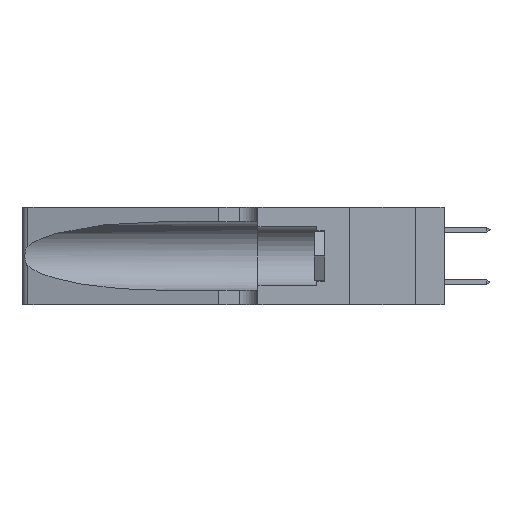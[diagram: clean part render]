
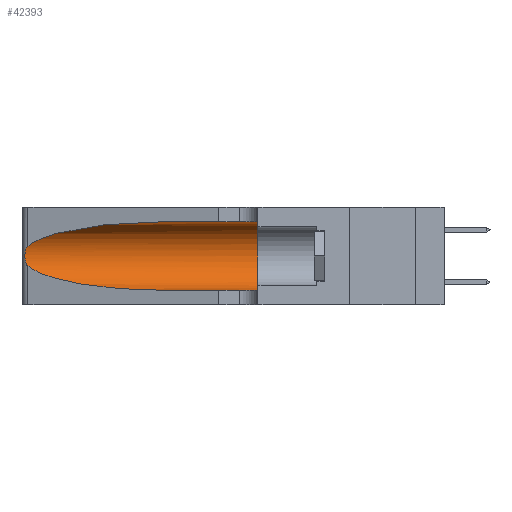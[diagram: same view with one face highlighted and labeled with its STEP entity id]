
A CAD part, left-side view. The second image highlights one B-rep face of the part: STEP entity #42393.
In plain terms, the highlighted cylindrical face has radius 3.308 mm (diameter 6.617 mm), a partial arc.
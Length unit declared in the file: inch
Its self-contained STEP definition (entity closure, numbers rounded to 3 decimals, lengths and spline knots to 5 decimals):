
#1410 = CARTESIAN_POINT ( 'NONE',  ( 0.26075, 1.23896, 0.178 ) ) ;
#1549 = CARTESIAN_POINT ( 'NONE',  ( 0.25854, 1.2359, 0.20912 ) ) ;
#2740 =( BOUNDED_CURVE ( )  B_SPLINE_CURVE ( 3, ( #5531, #25477, #35617, #6346 ),
 .UNSPECIFIED., .F., .F. ) 
 B_SPLINE_CURVE_WITH_KNOTS ( ( 4, 4 ),
 ( 1.5708, 2.84003 ),
 .UNSPECIFIED. ) 
 CURVE ( )  GEOMETRIC_REPRESENTATION_ITEM ( )  RATIONAL_B_SPLINE_CURVE ( ( 1., 0.87, 0.87, 1. ) ) 
 REPRESENTATION_ITEM ( '' )  );
#4674 = CARTESIAN_POINT ( 'NONE',  ( 0.25789, 1.23486, 0.15765 ) ) ;
#5241 = DIRECTION ( 'NONE',  ( 0., -1., 0. ) ) ;
#5279 = EDGE_CURVE ( 'NONE', #29261, #35275, #19362, .T. ) ;
#5531 = CARTESIAN_POINT ( 'NONE',  ( 0.1305, 0.72297, 0.31525 ) ) ;
#5534 = CARTESIAN_POINT ( 'NONE',  ( 0.1305, 1.61858, 0.185 ) ) ;
#6346 = CARTESIAN_POINT ( 'NONE',  ( 0.25487, 1.22718, 0.22369 ) ) ;
#7813 = CARTESIAN_POINT ( 'NONE',  ( 0.25856, 1.23593, 0.16098 ) ) ;
#8115 = CARTESIAN_POINT ( 'NONE',  ( 0.25555, 1.22994, 0.2215 ) ) ;
#9507 = ORIENTED_EDGE ( 'NONE', *, *, #23897, .T. ) ;
#10848 = B_SPLINE_CURVE_WITH_KNOTS ( 'NONE', 3,
 ( #21062, #8115, #34177, #40543, #1549, #24345, #31143, #1410, #24491, #7813, #4674, #30851, #27969, #20884 ),
 .UNSPECIFIED., .F., .F.,
 ( 4, 2, 2, 2, 2, 2, 4 ),
 ( 0., 0.00027, 0.00053, 0.00107, 0.0016, 0.00187, 0.00214 ),
 .UNSPECIFIED. ) ;
#11268 = DIRECTION ( 'NONE',  ( 0., 1., 0. ) ) ;
#11729 = CARTESIAN_POINT ( 'NONE',  ( 0.25487, 1.22718, 0.22369 ) ) ;
#13316 = EDGE_CURVE ( 'NONE', #35985, #35275, #42242, .T. ) ;
#14075 = CARTESIAN_POINT ( 'NONE',  ( 0.1305, 0.35, 0.05475 ) ) ;
#14426 = DIRECTION ( 'NONE',  ( 0., 0., 1. ) ) ;
#15005 = CARTESIAN_POINT ( 'NONE',  ( 0.1305, 1.61858, 0.31525 ) ) ;
#16209 = AXIS2_PLACEMENT_3D ( 'NONE', #5534, #18297, #28076 ) ;
#16345 = CARTESIAN_POINT ( 'NONE',  ( 0.1305, 0.72297, 0.05475 ) ) ;
#17850 = ORIENTED_EDGE ( 'NONE', *, *, #13316, .F. ) ;
#17932 = DIRECTION ( 'NONE',  ( 0., -1., 0. ) ) ;
#18297 = DIRECTION ( 'NONE',  ( 0., -1., 0. ) ) ;
#19362 = LINE ( 'NONE', #27725, #31795 ) ;
#20579 = CARTESIAN_POINT ( 'NONE',  ( 0.25487, 1.22718, 0.14631 ) ) ;
#20792 = ORIENTED_EDGE ( 'NONE', *, *, #36692, .T. ) ;
#20884 = CARTESIAN_POINT ( 'NONE',  ( 0.25487, 1.22718, 0.14631 ) ) ;
#21057 = AXIS2_PLACEMENT_3D ( 'NONE', #34164, #11268, #14426 ) ;
#21062 = CARTESIAN_POINT ( 'NONE',  ( 0.25487, 1.22718, 0.22369 ) ) ;
#21414 = CARTESIAN_POINT ( 'NONE',  ( 0.1305, 0.72297, 0.31525 ) ) ;
#21697 = CARTESIAN_POINT ( 'NONE',  ( 0.2373, 1.15595, 0.08982 ) ) ;
#22472 =( BOUNDED_CURVE ( )  B_SPLINE_CURVE ( 3, ( #41901, #21697, #38868, #16345 ),
 .UNSPECIFIED., .F., .F. ) 
 B_SPLINE_CURVE_WITH_KNOTS ( ( 4, 4 ),
 ( 3.44316, 4.71239 ),
 .UNSPECIFIED. ) 
 CURVE ( )  GEOMETRIC_REPRESENTATION_ITEM ( )  RATIONAL_B_SPLINE_CURVE ( ( 1., 0.87, 0.87, 1. ) ) 
 REPRESENTATION_ITEM ( '' )  );
#23897 = EDGE_CURVE ( 'NONE', #36550, #29261, #22472, .T. ) ;
#24345 = CARTESIAN_POINT ( 'NONE',  ( 0.26018, 1.23835, 0.19895 ) ) ;
#24491 = CARTESIAN_POINT ( 'NONE',  ( 0.26017, 1.23833, 0.17102 ) ) ;
#24804 = ORIENTED_EDGE ( 'NONE', *, *, #28854, .F. ) ;
#25477 = CARTESIAN_POINT ( 'NONE',  ( 0.18966, 0.96281, 0.31525 ) ) ;
#27725 = CARTESIAN_POINT ( 'NONE',  ( 0.1305, 1.61858, 0.05475 ) ) ;
#27969 = CARTESIAN_POINT ( 'NONE',  ( 0.25555, 1.22993, 0.14849 ) ) ;
#28076 = DIRECTION ( 'NONE',  ( 0., 0., -1. ) ) ;
#28854 = EDGE_CURVE ( 'NONE', #37371, #35985, #39731, .T. ) ;
#29261 = VERTEX_POINT ( 'NONE', #34269 ) ;
#29426 = CARTESIAN_POINT ( 'NONE',  ( 0.1305, 0.35, 0.31525 ) ) ;
#29814 = EDGE_CURVE ( 'NONE', #37371, #37535, #2740, .T. ) ;
#30851 = CARTESIAN_POINT ( 'NONE',  ( 0.25639, 1.23186, 0.15144 ) ) ;
#30926 = VECTOR ( 'NONE', #5241, 39.37008 ) ;
#31143 = CARTESIAN_POINT ( 'NONE',  ( 0.26075, 1.23896, 0.19203 ) ) ;
#31795 = VECTOR ( 'NONE', #17932, 39.37008 ) ;
#34164 = CARTESIAN_POINT ( 'NONE',  ( 0.1305, 0.35, 0.185 ) ) ;
#34177 = CARTESIAN_POINT ( 'NONE',  ( 0.25639, 1.23184, 0.21858 ) ) ;
#34269 = CARTESIAN_POINT ( 'NONE',  ( 0.1305, 0.72297, 0.05475 ) ) ;
#34827 = ORIENTED_EDGE ( 'NONE', *, *, #29814, .T. ) ;
#35275 = VERTEX_POINT ( 'NONE', #14075 ) ;
#35617 = CARTESIAN_POINT ( 'NONE',  ( 0.2373, 1.15595, 0.28018 ) ) ;
#35985 = VERTEX_POINT ( 'NONE', #29426 ) ;
#36550 = VERTEX_POINT ( 'NONE', #20579 ) ;
#36692 = EDGE_CURVE ( 'NONE', #37535, #36550, #10848, .T. ) ;
#36757 = EDGE_LOOP ( 'NONE', ( #34827, #20792, #9507, #40102, #17850, #24804 ) ) ;
#36830 = CYLINDRICAL_SURFACE ( 'NONE', #16209, 0.13025 ) ;
#37371 = VERTEX_POINT ( 'NONE', #21414 ) ;
#37535 = VERTEX_POINT ( 'NONE', #11729 ) ;
#38868 = CARTESIAN_POINT ( 'NONE',  ( 0.18966, 0.96281, 0.05475 ) ) ;
#39731 = LINE ( 'NONE', #15005, #30926 ) ;
#40102 = ORIENTED_EDGE ( 'NONE', *, *, #5279, .T. ) ;
#40543 = CARTESIAN_POINT ( 'NONE',  ( 0.25787, 1.23484, 0.2124 ) ) ;
#41039 = FACE_OUTER_BOUND ( 'NONE', #36757, .T. ) ;
#41901 = CARTESIAN_POINT ( 'NONE',  ( 0.25487, 1.22718, 0.14631 ) ) ;
#42242 = CIRCLE ( 'NONE', #21057, 0.13025 ) ;
#42393 = ADVANCED_FACE ( 'NONE', ( #41039 ), #36830, .F. ) ;
